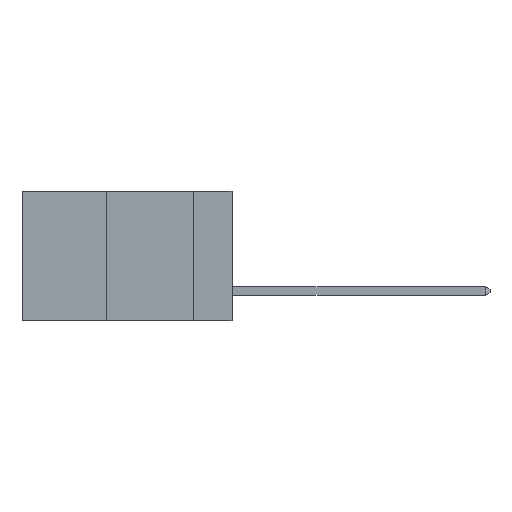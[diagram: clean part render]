
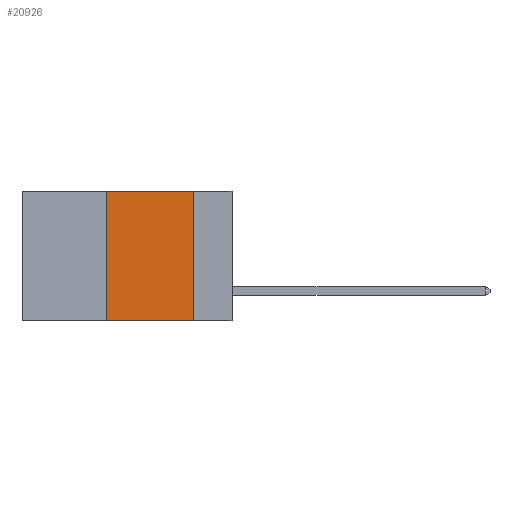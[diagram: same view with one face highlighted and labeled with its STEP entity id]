
A CAD part, left-side view. The second image highlights one B-rep face of the part: STEP entity #20926.
In plain terms, the highlighted planar face has unit normal (-1, 0, 0).
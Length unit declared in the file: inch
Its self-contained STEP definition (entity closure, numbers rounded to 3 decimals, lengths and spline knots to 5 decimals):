
#418 = CARTESIAN_POINT ( 'NONE',  ( 0., 0.11, -0.37 ) ) ;
#538 = FACE_OUTER_BOUND ( 'NONE', #9293, .T. ) ;
#1915 = CARTESIAN_POINT ( 'NONE',  ( 0., 0.6, -0.37 ) ) ;
#2768 = EDGE_CURVE ( 'NONE', #17790, #23519, #12181, .T. ) ;
#2880 = VERTEX_POINT ( 'NONE', #418 ) ;
#3727 = DIRECTION ( 'NONE',  ( 0., 0., -1. ) ) ;
#3729 = ORIENTED_EDGE ( 'NONE', *, *, #14351, .F. ) ;
#3955 = DIRECTION ( 'NONE',  ( 0., -1., 0. ) ) ;
#4208 = LINE ( 'NONE', #1915, #13959 ) ;
#4983 = ORIENTED_EDGE ( 'NONE', *, *, #14504, .T. ) ;
#5258 = LINE ( 'NONE', #15265, #24890 ) ;
#7923 = VECTOR ( 'NONE', #16589, 39.37008 ) ;
#9293 = EDGE_LOOP ( 'NONE', ( #23214, #3729, #21558, #4983 ) ) ;
#9440 = CARTESIAN_POINT ( 'NONE',  ( 0., 0.36, 0. ) ) ;
#9550 = DIRECTION ( 'NONE',  ( 0., 0., -1. ) ) ;
#12022 = CARTESIAN_POINT ( 'NONE',  ( 0., 0.36, 0. ) ) ;
#12181 = LINE ( 'NONE', #9440, #12794 ) ;
#12292 = CARTESIAN_POINT ( 'NONE',  ( 0., 0.36, -0.37 ) ) ;
#12569 = EDGE_CURVE ( 'NONE', #23750, #2880, #5258, .T. ) ;
#12794 = VECTOR ( 'NONE', #22714, 39.37008 ) ;
#12944 = CARTESIAN_POINT ( 'NONE',  ( 0., 0.6, 0. ) ) ;
#13478 = PLANE ( 'NONE',  #16838 ) ;
#13959 = VECTOR ( 'NONE', #3955, 39.37008 ) ;
#14351 = EDGE_CURVE ( 'NONE', #23519, #23750, #18154, .T. ) ;
#14504 = EDGE_CURVE ( 'NONE', #17790, #2880, #4208, .T. ) ;
#15265 = CARTESIAN_POINT ( 'NONE',  ( 0., 0.11, 0. ) ) ;
#15286 = CARTESIAN_POINT ( 'NONE',  ( 0., 0.6, 0. ) ) ;
#15369 = DIRECTION ( 'NONE',  ( 1., 0., 0. ) ) ;
#16589 = DIRECTION ( 'NONE',  ( 0., -1., 0. ) ) ;
#16838 = AXIS2_PLACEMENT_3D ( 'NONE', #15286, #15369, #3727 ) ;
#17790 = VERTEX_POINT ( 'NONE', #12292 ) ;
#18154 = LINE ( 'NONE', #12944, #7923 ) ;
#20926 = ADVANCED_FACE ( 'NONE', ( #538 ), #13478, .F. ) ;
#21558 = ORIENTED_EDGE ( 'NONE', *, *, #2768, .F. ) ;
#22714 = DIRECTION ( 'NONE',  ( 0., 0., 1. ) ) ;
#23214 = ORIENTED_EDGE ( 'NONE', *, *, #12569, .F. ) ;
#23519 = VERTEX_POINT ( 'NONE', #12022 ) ;
#23750 = VERTEX_POINT ( 'NONE', #23842 ) ;
#23842 = CARTESIAN_POINT ( 'NONE',  ( 0., 0.11, 0. ) ) ;
#24890 = VECTOR ( 'NONE', #9550, 39.37008 ) ;
